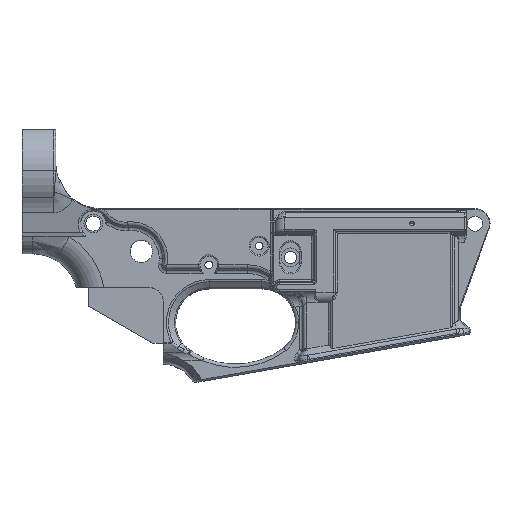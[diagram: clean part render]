
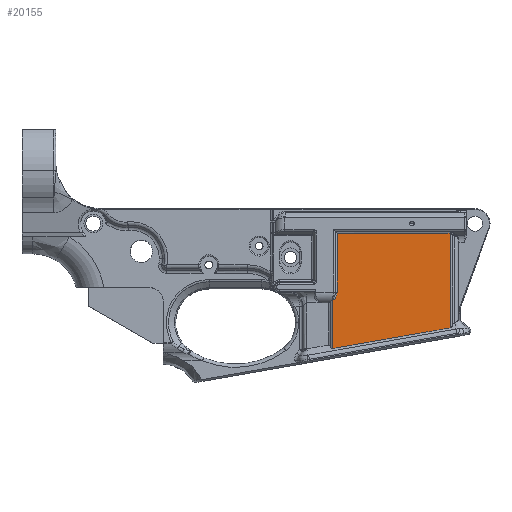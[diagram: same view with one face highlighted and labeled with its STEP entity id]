
A CAD part, top view. The second image highlights one B-rep face of the part: STEP entity #20155.
In plain terms, the highlighted planar face has unit normal (0, 0, 1).
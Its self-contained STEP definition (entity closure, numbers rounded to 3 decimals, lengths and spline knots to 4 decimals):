
#2346 = CARTESIAN_POINT ( 'NONE',  ( -2.3623, -1.274, 0.6325 ) ) ;
#2401 = B_SPLINE_CURVE_WITH_KNOTS ( 'NONE', 3,
 ( #42181, #25043, #30273, #2346, #36966, #42906 ),
 .UNSPECIFIED., .F., .F.,
 ( 4, 2, 4 ),
 ( 0., 0.0004, 0.0008 ),
 .UNSPECIFIED. ) ;
#5866 = CARTESIAN_POINT ( 'NONE',  ( -0.4173, -4.4545, 0.6325 ) ) ;
#6154 = DIRECTION ( 'NONE',  ( 0., 1., 0. ) ) ;
#8557 = ORIENTED_EDGE ( 'NONE', *, *, #22302, .T. ) ;
#10170 = ORIENTED_EDGE ( 'NONE', *, *, #24371, .T. ) ;
#11859 = ORIENTED_EDGE ( 'NONE', *, *, #67778, .T. ) ;
#13172 = CARTESIAN_POINT ( 'NONE',  ( -2.3442, -1.2641, 0.6325 ) ) ;
#14902 = PLANE ( 'NONE',  #73369 ) ;
#16799 =( BOUNDED_CURVE ( )  B_SPLINE_CURVE ( 3, ( #58923, #51892, #64165, #13172 ),
 .UNSPECIFIED., .F., .T. ) 
 B_SPLINE_CURVE_WITH_KNOTS ( ( 4, 4 ),
 ( 3.1416, 3.7456 ),
 .UNSPECIFIED. ) 
 CURVE ( )  GEOMETRIC_REPRESENTATION_ITEM ( )  RATIONAL_B_SPLINE_CURVE ( ( 1., 0.97, 0.97, 1. ) ) 
 REPRESENTATION_ITEM ( '' )  );
#17004 = LINE ( 'NONE', #5866, #59015 ) ;
#18129 = EDGE_LOOP ( 'NONE', ( #63894, #10170, #61630, #66136, #8557, #11859, #21100 ) ) ;
#20155 = ADVANCED_FACE ( 'NONE', ( #30965 ), #14902, .T. ) ;
#21100 = ORIENTED_EDGE ( 'NONE', *, *, #42125, .T. ) ;
#22302 = EDGE_CURVE ( 'NONE', #68612, #37954, #17004, .T. ) ;
#22970 = LINE ( 'NONE', #45707, #70773 ) ;
#23730 = VERTEX_POINT ( 'NONE', #48898 ) ;
#23794 = DIRECTION ( 'NONE',  ( 0.985, 0.174, 0. ) ) ;
#24012 = CARTESIAN_POINT ( 'NONE',  ( -0.4173, -0.1616, 0.6325 ) ) ;
#24371 = EDGE_CURVE ( 'NONE', #63609, #36365, #2401, .T. ) ;
#25043 = CARTESIAN_POINT ( 'NONE',  ( -2.3485, -1.267, 0.6325 ) ) ;
#28021 = EDGE_CURVE ( 'NONE', #52317, #63609, #16799, .T. ) ;
#30273 = CARTESIAN_POINT ( 'NONE',  ( -2.3529, -1.2697, 0.6325 ) ) ;
#30965 = FACE_OUTER_BOUND ( 'NONE', #18129, .T. ) ;
#33443 = DIRECTION ( 'NONE',  ( 0., 1., 0. ) ) ;
#35341 = EDGE_CURVE ( 'NONE', #23730, #68612, #47929, .T. ) ;
#35521 = VECTOR ( 'NONE', #23794, 39.3701 ) ;
#36272 = DIRECTION ( 'NONE',  ( 0., -1., 0. ) ) ;
#36365 = VERTEX_POINT ( 'NONE', #48066 ) ;
#36966 = CARTESIAN_POINT ( 'NONE',  ( -2.3672, -1.2755, 0.6325 ) ) ;
#37954 = VERTEX_POINT ( 'NONE', #24012 ) ;
#38848 = CARTESIAN_POINT ( 'NONE',  ( -2.3039, -0.1616, 0.6325 ) ) ;
#41785 = DIRECTION ( 'NONE',  ( 1., 0., 0. ) ) ;
#42125 = EDGE_CURVE ( 'NONE', #56558, #52317, #47096, .T. ) ;
#42181 = CARTESIAN_POINT ( 'NONE',  ( -2.3442, -1.2641, 0.6325 ) ) ;
#42248 = CARTESIAN_POINT ( 'NONE',  ( -2.3039, -1.1448, 0.6325 ) ) ;
#42906 = CARTESIAN_POINT ( 'NONE',  ( -2.3724, -1.2759, 0.6325 ) ) ;
#44337 = CARTESIAN_POINT ( 'NONE',  ( -0.4173, -1.7416, 0.6325 ) ) ;
#45707 = CARTESIAN_POINT ( 'NONE',  ( -2.3239, -0.1616, 0.6325 ) ) ;
#45960 = VECTOR ( 'NONE', #6154, 39.3701 ) ;
#47096 = LINE ( 'NONE', #69771, #69734 ) ;
#47929 = LINE ( 'NONE', #58732, #35521 ) ;
#48066 = CARTESIAN_POINT ( 'NONE',  ( -2.3724, -1.2759, 0.6325 ) ) ;
#48898 = CARTESIAN_POINT ( 'NONE',  ( -2.3724, -2.0863, 0.6325 ) ) ;
#50824 = LINE ( 'NONE', #63095, #45960 ) ;
#50988 = EDGE_CURVE ( 'NONE', #23730, #36365, #50824, .T. ) ;
#51892 = CARTESIAN_POINT ( 'NONE',  ( -2.3039, -1.1877, 0.6325 ) ) ;
#52317 = VERTEX_POINT ( 'NONE', #42248 ) ;
#56287 = CARTESIAN_POINT ( 'NONE',  ( -2.3442, -1.2641, 0.6325 ) ) ;
#56558 = VERTEX_POINT ( 'NONE', #38848 ) ;
#58732 = CARTESIAN_POINT ( 'NONE',  ( -2.7774, -2.1577, 0.6325 ) ) ;
#58923 = CARTESIAN_POINT ( 'NONE',  ( -2.3039, -1.1448, 0.6325 ) ) ;
#59015 = VECTOR ( 'NONE', #33443, 39.3701 ) ;
#61630 = ORIENTED_EDGE ( 'NONE', *, *, #50988, .F. ) ;
#63095 = CARTESIAN_POINT ( 'NONE',  ( -2.3724, -4.4545, 0.6325 ) ) ;
#63609 = VERTEX_POINT ( 'NONE', #56287 ) ;
#63894 = ORIENTED_EDGE ( 'NONE', *, *, #28021, .T. ) ;
#64165 = CARTESIAN_POINT ( 'NONE',  ( -2.3178, -1.2287, 0.6325 ) ) ;
#64449 = DIRECTION ( 'NONE',  ( 0., 0., 1. ) ) ;
#65182 = CARTESIAN_POINT ( 'NONE',  ( -2.3724, -4.4545, 0.6325 ) ) ;
#66136 = ORIENTED_EDGE ( 'NONE', *, *, #35341, .T. ) ;
#67778 = EDGE_CURVE ( 'NONE', #37954, #56558, #22970, .T. ) ;
#68372 = DIRECTION ( 'NONE',  ( -1., 0., 0. ) ) ;
#68612 = VERTEX_POINT ( 'NONE', #44337 ) ;
#69734 = VECTOR ( 'NONE', #36272, 39.3701 ) ;
#69771 = CARTESIAN_POINT ( 'NONE',  ( -2.3039, -1.1448, 0.6325 ) ) ;
#70773 = VECTOR ( 'NONE', #68372, 39.3701 ) ;
#73369 = AXIS2_PLACEMENT_3D ( 'NONE', #65182, #64449, #41785 ) ;
